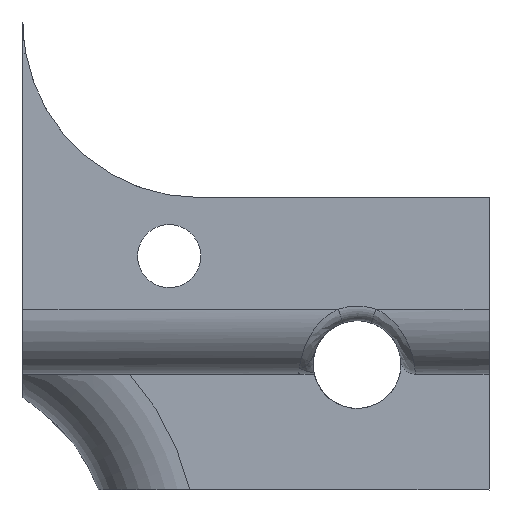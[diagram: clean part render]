
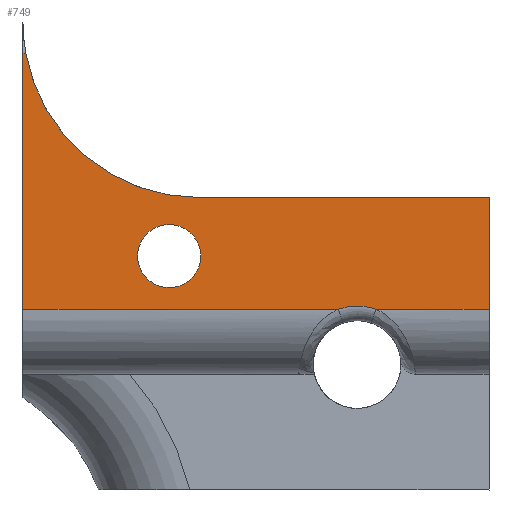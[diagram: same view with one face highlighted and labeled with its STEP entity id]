
A CAD part, left-side view. The second image highlights one B-rep face of the part: STEP entity #749.
In plain terms, the highlighted planar face has unit normal (-1, 0, 0).
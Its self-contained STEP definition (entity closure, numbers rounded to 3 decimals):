
#26 = VERTEX_POINT ( 'NONE', #2669 ) ;
#108 = ORIENTED_EDGE ( 'NONE', *, *, #2789, .F. ) ;
#147 = CARTESIAN_POINT ( 'NONE',  ( -5.851, 50.479, 152.857 ) ) ;
#192 = CARTESIAN_POINT ( 'NONE',  ( -5.851, -111.446, 159.219 ) ) ;
#234 = DIRECTION ( 'NONE',  ( -1., 0., 0. ) ) ;
#237 = VERTEX_POINT ( 'NONE', #1874 ) ;
#241 = DIRECTION ( 'NONE',  ( 0., 1., 0. ) ) ;
#320 = VECTOR ( 'NONE', #241, 1000. ) ;
#355 = VECTOR ( 'NONE', #2547, 1000. ) ;
#357 = CARTESIAN_POINT ( 'NONE',  ( -5.851, 66.047, 174.861 ) ) ;
#480 = DIRECTION ( 'NONE',  ( 0., -1., 0. ) ) ;
#545 = CARTESIAN_POINT ( 'NONE',  ( -5.851, 15.761, 159.219 ) ) ;
#605 = VECTOR ( 'NONE', #3046, 1000. ) ;
#606 = CARTESIAN_POINT ( 'NONE',  ( -5.851, 66.354, 174.861 ) ) ;
#611 = VERTEX_POINT ( 'NONE', #1605 ) ;
#649 = VERTEX_POINT ( 'NONE', #910 ) ;
#674 = VERTEX_POINT ( 'NONE', #545 ) ;
#738 = CARTESIAN_POINT ( 'NONE',  ( -5.851, 47.304, 178.269 ) ) ;
#749 = ADVANCED_FACE ( 'NONE', ( #2928, #2023 ), #4096, .T. ) ;
#810 = CARTESIAN_POINT ( 'NONE',  ( -5.851, 47.304, 159.219 ) ) ;
#827 = CARTESIAN_POINT ( 'NONE',  ( -5.851, 29.388, 147.434 ) ) ;
#903 = ORIENTED_EDGE ( 'NONE', *, *, #3808, .T. ) ;
#905 = CARTESIAN_POINT ( 'NONE',  ( -5.851, 312.963, 174.861 ) ) ;
#910 = CARTESIAN_POINT ( 'NONE',  ( -5.851, 28.05, 147.1 ) ) ;
#932 = VERTEX_POINT ( 'NONE', #810 ) ;
#946 = VERTEX_POINT ( 'NONE', #606 ) ;
#1012 = VECTOR ( 'NONE', #3330, 1000. ) ;
#1099 = DIRECTION ( 'NONE',  ( 0., 0., 1. ) ) ;
#1103 = DIRECTION ( 'NONE',  ( -1., 0., 0. ) ) ;
#1188 = CARTESIAN_POINT ( 'NONE',  ( -5.851, 28.05, 147.1 ) ) ;
#1219 = AXIS2_PLACEMENT_3D ( 'NONE', #2270, #234, #2587 ) ;
#1227 = ORIENTED_EDGE ( 'NONE', *, *, #1565, .F. ) ;
#1233 = ORIENTED_EDGE ( 'NONE', *, *, #3052, .T. ) ;
#1250 = DIRECTION ( 'NONE',  ( 0., 0., 1. ) ) ;
#1415 = ORIENTED_EDGE ( 'NONE', *, *, #2735, .F. ) ;
#1422 = VERTEX_POINT ( 'NONE', #3421 ) ;
#1565 = EDGE_CURVE ( 'NONE', #674, #1422, #3227, .T. ) ;
#1605 = CARTESIAN_POINT ( 'NONE',  ( -5.851, 32.116, 147.1 ) ) ;
#1631 = EDGE_CURVE ( 'NONE', #237, #611, #2803, .T. ) ;
#1730 = LINE ( 'NONE', #3579, #4290 ) ;
#1782 = AXIS2_PLACEMENT_3D ( 'NONE', #738, #3092, #1099 ) ;
#1874 = CARTESIAN_POINT ( 'NONE',  ( -5.851, 66.354, 147.1 ) ) ;
#2023 = FACE_BOUND ( 'NONE', #4126, .T. ) ;
#2079 = ORIENTED_EDGE ( 'NONE', *, *, #2239, .T. ) ;
#2176 = CARTESIAN_POINT ( 'NONE',  ( -5.851, 32.116, 147.1 ) ) ;
#2177 = LINE ( 'NONE', #192, #355 ) ;
#2239 = EDGE_CURVE ( 'NONE', #3786, #946, #3920, .T. ) ;
#2270 = CARTESIAN_POINT ( 'NONE',  ( -5.851, 50.479, 152.857 ) ) ;
#2306 = ORIENTED_EDGE ( 'NONE', *, *, #1631, .T. ) ;
#2430 = ORIENTED_EDGE ( 'NONE', *, *, #3341, .T. ) ;
#2499 = DIRECTION ( 'NONE',  ( -1., 0., 0. ) ) ;
#2547 = DIRECTION ( 'NONE',  ( 0., -1., 0. ) ) ;
#2587 = DIRECTION ( 'NONE',  ( 0., -1., 0. ) ) ;
#2657 = EDGE_CURVE ( 'NONE', #2835, #26, #3946, .T. ) ;
#2669 = CARTESIAN_POINT ( 'NONE',  ( -5.851, 53.908, 152.857 ) ) ;
#2735 = EDGE_CURVE ( 'NONE', #932, #674, #2177, .T. ) ;
#2789 = EDGE_CURVE ( 'NONE', #237, #946, #1730, .T. ) ;
#2803 = LINE ( 'NONE', #3354, #1012 ) ;
#2815 = EDGE_CURVE ( 'NONE', #26, #2835, #3399, .T. ) ;
#2834 = CARTESIAN_POINT ( 'NONE',  ( -5.851, -89.942, 147.1 ) ) ;
#2835 = VERTEX_POINT ( 'NONE', #3587 ) ;
#2849 = CARTESIAN_POINT ( 'NONE',  ( -5.851, 30.778, 147.434 ) ) ;
#2924 = VECTOR ( 'NONE', #3784, 1000. ) ;
#2928 = FACE_OUTER_BOUND ( 'NONE', #4185, .T. ) ;
#3046 = DIRECTION ( 'NONE',  ( 0., -1., 0. ) ) ;
#3052 = EDGE_CURVE ( 'NONE', #611, #649, #3431, .T. ) ;
#3092 = DIRECTION ( 'NONE',  ( 1., 0., 0. ) ) ;
#3171 = CARTESIAN_POINT ( 'NONE',  ( -5.851, 28.71, 147.323 ) ) ;
#3227 = LINE ( 'NONE', #3807, #2924 ) ;
#3293 = AXIS2_PLACEMENT_3D ( 'NONE', #147, #2499, #480 ) ;
#3324 = ORIENTED_EDGE ( 'NONE', *, *, #2657, .F. ) ;
#3326 = CIRCLE ( 'NONE', #1782, 19.05 ) ;
#3330 = DIRECTION ( 'NONE',  ( 0., -1., 0. ) ) ;
#3341 = EDGE_CURVE ( 'NONE', #932, #3786, #3326, .T. ) ;
#3354 = CARTESIAN_POINT ( 'NONE',  ( -5.851, -89.942, 147.1 ) ) ;
#3391 = AXIS2_PLACEMENT_3D ( 'NONE', #2834, #1103, #3428 ) ;
#3399 = CIRCLE ( 'NONE', #1219, 3.429 ) ;
#3421 = CARTESIAN_POINT ( 'NONE',  ( -5.851, 15.761, 147.1 ) ) ;
#3428 = DIRECTION ( 'NONE',  ( 0., -1., 0. ) ) ;
#3431 = B_SPLINE_CURVE_WITH_KNOTS ( 'NONE', 3,
 ( #2176, #4165, #2849, #827, #3171, #1188 ),
 .UNSPECIFIED., .F., .F.,
 ( 4, 2, 4 ),
 ( 0., 0.5, 1. ),
 .UNSPECIFIED. ) ;
#3579 = CARTESIAN_POINT ( 'NONE',  ( -5.851, 66.354, 147.1 ) ) ;
#3587 = CARTESIAN_POINT ( 'NONE',  ( -5.851, 47.05, 152.857 ) ) ;
#3784 = DIRECTION ( 'NONE',  ( 0., 0., -1. ) ) ;
#3786 = VERTEX_POINT ( 'NONE', #357 ) ;
#3807 = CARTESIAN_POINT ( 'NONE',  ( -5.851, 15.761, 147.1 ) ) ;
#3808 = EDGE_CURVE ( 'NONE', #649, #1422, #4047, .T. ) ;
#3920 = LINE ( 'NONE', #905, #320 ) ;
#3946 = CIRCLE ( 'NONE', #3293, 3.429 ) ;
#4033 = CARTESIAN_POINT ( 'NONE',  ( -5.851, -89.942, 147.1 ) ) ;
#4047 = LINE ( 'NONE', #4033, #605 ) ;
#4096 = PLANE ( 'NONE',  #3391 ) ;
#4126 = EDGE_LOOP ( 'NONE', ( #3324, #4198 ) ) ;
#4165 = CARTESIAN_POINT ( 'NONE',  ( -5.851, 31.456, 147.322 ) ) ;
#4185 = EDGE_LOOP ( 'NONE', ( #1227, #1415, #2430, #2079, #108, #2306, #1233, #903 ) ) ;
#4198 = ORIENTED_EDGE ( 'NONE', *, *, #2815, .F. ) ;
#4290 = VECTOR ( 'NONE', #1250, 1000. ) ;
